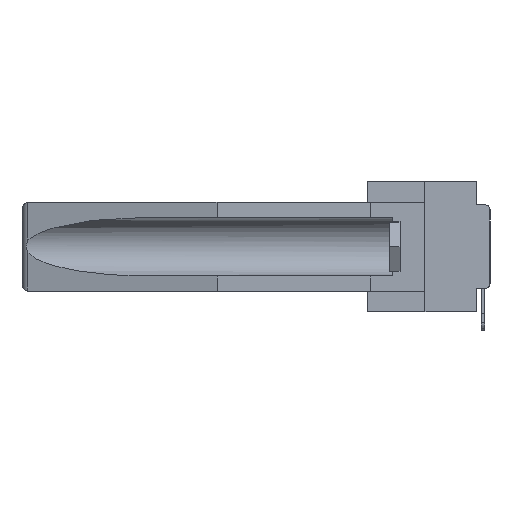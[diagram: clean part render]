
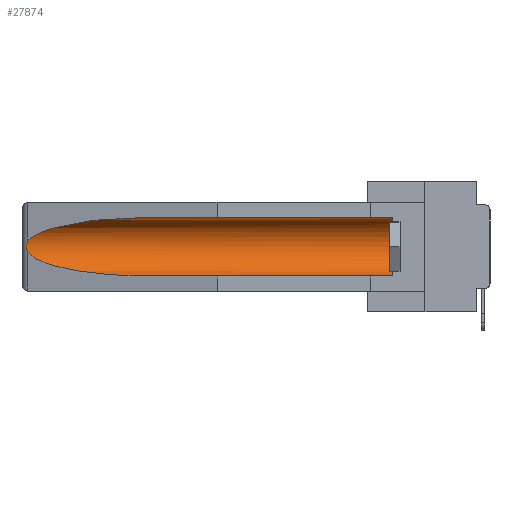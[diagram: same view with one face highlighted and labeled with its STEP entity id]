
A CAD part, left-side view. The second image highlights one B-rep face of the part: STEP entity #27874.
In plain terms, the highlighted cylindrical face has radius 2.857 mm (diameter 5.715 mm), a partial arc.
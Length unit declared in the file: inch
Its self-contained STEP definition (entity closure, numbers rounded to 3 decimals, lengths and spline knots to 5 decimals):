
#10 = CARTESIAN_POINT ( 'NONE',  ( 0.2675, 1.53308, -0.16763 ) ) ;
#728 = CARTESIAN_POINT ( 'NONE',  ( 0.155, 0.126, -0.059 ) ) ;
#2948 = VECTOR ( 'NONE', #3806, 39.37008 ) ;
#3142 = CARTESIAN_POINT ( 'NONE',  ( 0.155, 1.07973, -0.284 ) ) ;
#3324 = CARTESIAN_POINT ( 'NONE',  ( 0.26655, 1.53094, -0.18657 ) ) ;
#3326 = EDGE_CURVE ( 'NONE', #21322, #30847, #34449, .T. ) ;
#3517 = CARTESIAN_POINT ( 'NONE',  ( 0.26537, 1.52718, -0.19328 ) ) ;
#3806 = DIRECTION ( 'NONE',  ( 0., 1., 0. ) ) ;
#5299 = CYLINDRICAL_SURFACE ( 'NONE', #32614, 0.1125 ) ;
#6515 =( BOUNDED_CURVE ( )  B_SPLINE_CURVE ( 3, ( #10920, #17380, #30846, #3142 ),
 .UNSPECIFIED., .F., .F. ) 
 B_SPLINE_CURVE_WITH_KNOTS ( ( 4, 4 ),
 ( 0.1948, 1.5708 ),
 .UNSPECIFIED. ) 
 CURVE ( )  GEOMETRIC_REPRESENTATION_ITEM ( )  RATIONAL_B_SPLINE_CURVE ( ( 1., 0.848, 0.848, 1. ) ) 
 REPRESENTATION_ITEM ( '' )  );
#6578 = CARTESIAN_POINT ( 'NONE',  ( 0.155, -0.30754, -0.059 ) ) ;
#7680 = CARTESIAN_POINT ( 'NONE',  ( 0.21114, 1.30732, -0.059 ) ) ;
#7968 = VERTEX_POINT ( 'NONE', #728 ) ;
#8150 = ORIENTED_EDGE ( 'NONE', *, *, #27319, .F. ) ;
#8492 = CARTESIAN_POINT ( 'NONE',  ( 0.26597, 1.52961, -0.15275 ) ) ;
#8757 = CARTESIAN_POINT ( 'NONE',  ( 0.26537, 1.52718, -0.19328 ) ) ;
#8874 = CARTESIAN_POINT ( 'NONE',  ( 0.2673, 1.53269, -0.17917 ) ) ;
#9582 = EDGE_CURVE ( 'NONE', #7968, #24828, #29639, .T. ) ;
#10140 = CARTESIAN_POINT ( 'NONE',  ( 0.26537, 1.52718, -0.14972 ) ) ;
#10320 = AXIS2_PLACEMENT_3D ( 'NONE', #13393, #36081, #16165 ) ;
#10920 = CARTESIAN_POINT ( 'NONE',  ( 0.26537, 1.52718, -0.19328 ) ) ;
#10979 = ORIENTED_EDGE ( 'NONE', *, *, #30713, .T. ) ;
#11435 = CARTESIAN_POINT ( 'NONE',  ( 0.155, 1.07973, -0.284 ) ) ;
#11455 = CARTESIAN_POINT ( 'NONE',  ( 0.26537, 1.52718, -0.14972 ) ) ;
#12052 = EDGE_LOOP ( 'NONE', ( #10979, #15340, #22393, #8150, #19477, #28482 ) ) ;
#13393 = CARTESIAN_POINT ( 'NONE',  ( 0.155, 0.126, -0.1715 ) ) ;
#14450 = CIRCLE ( 'NONE', #10320, 0.1125 ) ;
#15340 = ORIENTED_EDGE ( 'NONE', *, *, #3326, .T. ) ;
#15869 = CARTESIAN_POINT ( 'NONE',  ( 0.155, 1.07973, -0.059 ) ) ;
#16165 = DIRECTION ( 'NONE',  ( 0., 0., 1. ) ) ;
#16393 = DIRECTION ( 'NONE',  ( 0., 0., 1. ) ) ;
#16528 = CARTESIAN_POINT ( 'NONE',  ( 0.155, -0.30754, -0.284 ) ) ;
#16544 = CARTESIAN_POINT ( 'NONE',  ( 0.25451, 1.48313, -0.09465 ) ) ;
#16697 = VECTOR ( 'NONE', #27759, 39.37008 ) ;
#17380 = CARTESIAN_POINT ( 'NONE',  ( 0.25451, 1.48313, -0.24835 ) ) ;
#19411 = VERTEX_POINT ( 'NONE', #27198 ) ;
#19477 = ORIENTED_EDGE ( 'NONE', *, *, #29634, .T. ) ;
#19514 = DIRECTION ( 'NONE',  ( 0., 1., 0. ) ) ;
#19762 = CARTESIAN_POINT ( 'NONE',  ( 0.26597, 1.5296, -0.19026 ) ) ;
#20634 =( BOUNDED_CURVE ( )  B_SPLINE_CURVE ( 3, ( #30368, #7680, #16544, #32955 ),
 .UNSPECIFIED., .F., .F. ) 
 B_SPLINE_CURVE_WITH_KNOTS ( ( 4, 4 ),
 ( 4.71239, 6.08839 ),
 .UNSPECIFIED. ) 
 CURVE ( )  GEOMETRIC_REPRESENTATION_ITEM ( )  RATIONAL_B_SPLINE_CURVE ( ( 1., 0.848, 0.848, 1. ) ) 
 REPRESENTATION_ITEM ( '' )  );
#20959 = EDGE_CURVE ( 'NONE', #30847, #30036, #6515, .T. ) ;
#21322 = VERTEX_POINT ( 'NONE', #10140 ) ;
#22393 = ORIENTED_EDGE ( 'NONE', *, *, #20959, .T. ) ;
#22518 = CARTESIAN_POINT ( 'NONE',  ( 0.2675, 1.53308, -0.17534 ) ) ;
#24828 = VERTEX_POINT ( 'NONE', #15869 ) ;
#25287 = CARTESIAN_POINT ( 'NONE',  ( 0.2673, 1.5327, -0.16383 ) ) ;
#27198 = CARTESIAN_POINT ( 'NONE',  ( 0.155, 0.126, -0.284 ) ) ;
#27319 = EDGE_CURVE ( 'NONE', #19411, #30036, #30896, .T. ) ;
#27759 = DIRECTION ( 'NONE',  ( 0., 1., 0. ) ) ;
#27874 = ADVANCED_FACE ( 'NONE', ( #33349 ), #5299, .F. ) ;
#28482 = ORIENTED_EDGE ( 'NONE', *, *, #9582, .T. ) ;
#28794 = CARTESIAN_POINT ( 'NONE',  ( 0.26654, 1.53092, -0.15636 ) ) ;
#29634 = EDGE_CURVE ( 'NONE', #19411, #7968, #14450, .T. ) ;
#29639 = LINE ( 'NONE', #6578, #2948 ) ;
#30036 = VERTEX_POINT ( 'NONE', #11435 ) ;
#30368 = CARTESIAN_POINT ( 'NONE',  ( 0.155, 1.07973, -0.059 ) ) ;
#30713 = EDGE_CURVE ( 'NONE', #24828, #21322, #20634, .T. ) ;
#30846 = CARTESIAN_POINT ( 'NONE',  ( 0.21114, 1.30732, -0.284 ) ) ;
#30847 = VERTEX_POINT ( 'NONE', #8757 ) ;
#30896 = LINE ( 'NONE', #16528, #16697 ) ;
#32614 = AXIS2_PLACEMENT_3D ( 'NONE', #36117, #19514, #16393 ) ;
#32955 = CARTESIAN_POINT ( 'NONE',  ( 0.26537, 1.52718, -0.14972 ) ) ;
#33349 = FACE_OUTER_BOUND ( 'NONE', #12052, .T. ) ;
#34449 = B_SPLINE_CURVE_WITH_KNOTS ( 'NONE', 3,
 ( #11455, #8492, #28794, #25287, #10, #22518, #8874, #3324, #19762, #3517 ),
 .UNSPECIFIED., .F., .F.,
 ( 4, 2, 2, 2, 4 ),
 ( 0., 0.00029, 0.00058, 0.00087, 0.00117 ),
 .UNSPECIFIED. ) ;
#36081 = DIRECTION ( 'NONE',  ( 0., -1., 0. ) ) ;
#36117 = CARTESIAN_POINT ( 'NONE',  ( 0.155, -0.30754, -0.1715 ) ) ;
